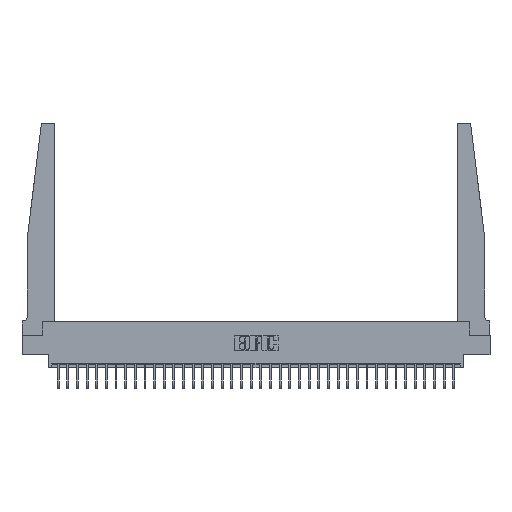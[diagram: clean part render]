
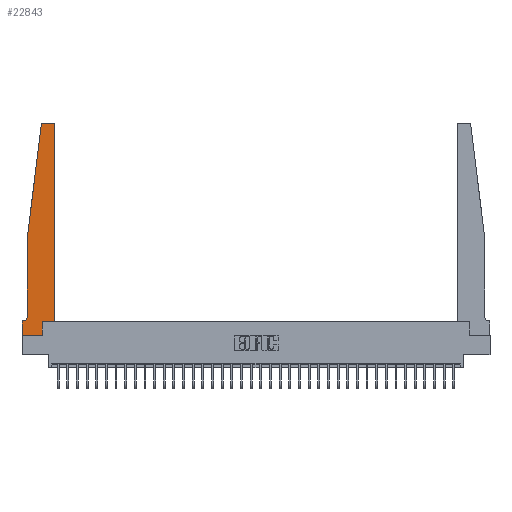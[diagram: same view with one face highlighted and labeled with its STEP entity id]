
A CAD part, top view. The second image highlights one B-rep face of the part: STEP entity #22843.
In plain terms, the highlighted planar face has unit normal (0, 0, 1).
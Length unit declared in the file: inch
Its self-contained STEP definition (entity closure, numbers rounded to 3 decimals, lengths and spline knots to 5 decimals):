
#201 = VECTOR ( 'NONE', #10803, 39.37008 ) ;
#574 = ORIENTED_EDGE ( 'NONE', *, *, #1850, .T. ) ;
#612 = CARTESIAN_POINT ( 'NONE',  ( 0., 0.1875, 0.37 ) ) ;
#661 = VERTEX_POINT ( 'NONE', #26374 ) ;
#939 = EDGE_CURVE ( 'NONE', #25772, #4605, #27736, .T. ) ;
#1061 = VECTOR ( 'NONE', #14592, 39.37008 ) ;
#1391 = DIRECTION ( 'NONE',  ( -0.122, -0.992, 0. ) ) ;
#1759 = LINE ( 'NONE', #13193, #201 ) ;
#1850 = EDGE_CURVE ( 'NONE', #4605, #10589, #10874, .T. ) ;
#2336 = VERTEX_POINT ( 'NONE', #3554 ) ;
#2435 = CARTESIAN_POINT ( 'NONE',  ( 0.425, 2.72, 0.37 ) ) ;
#2835 = CARTESIAN_POINT ( 'NONE',  ( 0.2605, 0., 0.37 ) ) ;
#2885 = AXIS2_PLACEMENT_3D ( 'NONE', #16379, #8387, #9315 ) ;
#3554 = CARTESIAN_POINT ( 'NONE',  ( 0., 0.1875, 0.37 ) ) ;
#3616 = AXIS2_PLACEMENT_3D ( 'NONE', #612, #29419, #15110 ) ;
#4387 = CARTESIAN_POINT ( 'NONE',  ( 0.425, 0.18, 0.37 ) ) ;
#4605 = VERTEX_POINT ( 'NONE', #12611 ) ;
#4637 = EDGE_CURVE ( 'NONE', #10589, #21681, #5285, .T. ) ;
#5099 = ORIENTED_EDGE ( 'NONE', *, *, #11352, .T. ) ;
#5236 = VECTOR ( 'NONE', #1391, 39.37008 ) ;
#5285 = LINE ( 'NONE', #15131, #16559 ) ;
#6821 = DIRECTION ( 'NONE',  ( 1., 0., 0. ) ) ;
#7274 = EDGE_CURVE ( 'NONE', #15423, #25772, #1759, .T. ) ;
#7332 = DIRECTION ( 'NONE',  ( 0., 1., 0. ) ) ;
#7657 = ORIENTED_EDGE ( 'NONE', *, *, #19373, .T. ) ;
#7843 = EDGE_LOOP ( 'NONE', ( #12732, #8987, #574, #9527, #17764, #7657, #10773, #11296, #29044, #15401, #5099, #12752 ) ) ;
#8076 = CARTESIAN_POINT ( 'NONE',  ( 0., 0., 0.37 ) ) ;
#8387 = DIRECTION ( 'NONE',  ( 0., 0., 1. ) ) ;
#8396 = VECTOR ( 'NONE', #28229, 39.37008 ) ;
#8714 = CARTESIAN_POINT ( 'NONE',  ( 0.425, 0.18, 0.37 ) ) ;
#8987 = ORIENTED_EDGE ( 'NONE', *, *, #939, .T. ) ;
#9048 = LINE ( 'NONE', #8076, #21014 ) ;
#9315 = DIRECTION ( 'NONE',  ( 1., 0., 0. ) ) ;
#9527 = ORIENTED_EDGE ( 'NONE', *, *, #4637, .T. ) ;
#9696 = CARTESIAN_POINT ( 'NONE',  ( 0.065, 0.1875, 0.37 ) ) ;
#9762 = VECTOR ( 'NONE', #7332, 39.37008 ) ;
#10589 = VERTEX_POINT ( 'NONE', #15959 ) ;
#10747 = EDGE_CURVE ( 'NONE', #10831, #15423, #12923, .T. ) ;
#10773 = ORIENTED_EDGE ( 'NONE', *, *, #18360, .T. ) ;
#10803 = DIRECTION ( 'NONE',  ( -1., 0., 0. ) ) ;
#10831 = VERTEX_POINT ( 'NONE', #2435 ) ;
#10874 = LINE ( 'NONE', #25245, #5236 ) ;
#11259 = AXIS2_PLACEMENT_3D ( 'NONE', #14144, #30876, #16585 ) ;
#11296 = ORIENTED_EDGE ( 'NONE', *, *, #23495, .T. ) ;
#11330 = CARTESIAN_POINT ( 'NONE',  ( 0.015, 0.2375, 0.37 ) ) ;
#11352 = EDGE_CURVE ( 'NONE', #18497, #10831, #20367, .T. ) ;
#12061 = CARTESIAN_POINT ( 'NONE',  ( 0.2605, 0.18, 0.37 ) ) ;
#12611 = CARTESIAN_POINT ( 'NONE',  ( 0.24675, 2.72367, 0.37 ) ) ;
#12732 = ORIENTED_EDGE ( 'NONE', *, *, #7274, .T. ) ;
#12752 = ORIENTED_EDGE ( 'NONE', *, *, #10747, .T. ) ;
#12923 = CIRCLE ( 'NONE', #11259, 0.03 ) ;
#13193 = CARTESIAN_POINT ( 'NONE',  ( 0.25, 2.75, 0.37 ) ) ;
#13413 = CARTESIAN_POINT ( 'NONE',  ( 0.27653, 2.75, 0.37 ) ) ;
#13713 = DIRECTION ( 'NONE',  ( -1., 0., 0. ) ) ;
#13905 = CARTESIAN_POINT ( 'NONE',  ( 0.425, 0.18, 0.37 ) ) ;
#14144 = CARTESIAN_POINT ( 'NONE',  ( 0.395, 2.72, 0.37 ) ) ;
#14592 = DIRECTION ( 'NONE',  ( -1., 0., 0. ) ) ;
#14847 = CARTESIAN_POINT ( 'NONE',  ( 0.065, 0.2375, 0.37 ) ) ;
#15110 = DIRECTION ( 'NONE',  ( 1., 0., 0. ) ) ;
#15131 = CARTESIAN_POINT ( 'NONE',  ( 0.065, 1.25, 0.37 ) ) ;
#15298 = DIRECTION ( 'NONE',  ( 0., -1., 0. ) ) ;
#15401 = ORIENTED_EDGE ( 'NONE', *, *, #16557, .T. ) ;
#15423 = VERTEX_POINT ( 'NONE', #23935 ) ;
#15959 = CARTESIAN_POINT ( 'NONE',  ( 0.065, 1.25, 0.37 ) ) ;
#16127 = VERTEX_POINT ( 'NONE', #2835 ) ;
#16379 = CARTESIAN_POINT ( 'NONE',  ( 0.27653, 2.72, 0.37 ) ) ;
#16467 = EDGE_CURVE ( 'NONE', #21681, #661, #29424, .T. ) ;
#16557 = EDGE_CURVE ( 'NONE', #19969, #18497, #28678, .T. ) ;
#16559 = VECTOR ( 'NONE', #17546, 39.37008 ) ;
#16585 = DIRECTION ( 'NONE',  ( 1., 0., 0. ) ) ;
#17032 = VERTEX_POINT ( 'NONE', #25702 ) ;
#17107 = LINE ( 'NONE', #29488, #22697 ) ;
#17546 = DIRECTION ( 'NONE',  ( 0., -1., 0. ) ) ;
#17764 = ORIENTED_EDGE ( 'NONE', *, *, #16467, .T. ) ;
#18360 = EDGE_CURVE ( 'NONE', #2336, #17032, #9048, .T. ) ;
#18497 = VERTEX_POINT ( 'NONE', #8714 ) ;
#18782 = EDGE_CURVE ( 'NONE', #16127, #19969, #21730, .T. ) ;
#18917 = FACE_OUTER_BOUND ( 'NONE', #7843, .T. ) ;
#19349 = VECTOR ( 'NONE', #6821, 39.37008 ) ;
#19373 = EDGE_CURVE ( 'NONE', #661, #2336, #25043, .T. ) ;
#19773 = AXIS2_PLACEMENT_3D ( 'NONE', #11330, #28028, #13713 ) ;
#19969 = VERTEX_POINT ( 'NONE', #12061 ) ;
#20367 = LINE ( 'NONE', #13905, #8396 ) ;
#21014 = VECTOR ( 'NONE', #15298, 39.37008 ) ;
#21650 = CARTESIAN_POINT ( 'NONE',  ( 0.2605, 0.18, 0.37 ) ) ;
#21681 = VERTEX_POINT ( 'NONE', #14847 ) ;
#21730 = LINE ( 'NONE', #21650, #9762 ) ;
#22697 = VECTOR ( 'NONE', #24676, 39.37008 ) ;
#22843 = ADVANCED_FACE ( 'NONE', ( #18917 ), #24609, .T. ) ;
#23495 = EDGE_CURVE ( 'NONE', #17032, #16127, #17107, .T. ) ;
#23935 = CARTESIAN_POINT ( 'NONE',  ( 0.395, 2.75, 0.37 ) ) ;
#24609 = PLANE ( 'NONE',  #3616 ) ;
#24676 = DIRECTION ( 'NONE',  ( 1., 0., 0. ) ) ;
#25043 = LINE ( 'NONE', #9696, #1061 ) ;
#25245 = CARTESIAN_POINT ( 'NONE',  ( 0.065, 1.25, 0.37 ) ) ;
#25702 = CARTESIAN_POINT ( 'NONE',  ( 0., 0., 0.37 ) ) ;
#25772 = VERTEX_POINT ( 'NONE', #13413 ) ;
#26374 = CARTESIAN_POINT ( 'NONE',  ( 0.015, 0.1875, 0.37 ) ) ;
#27736 = CIRCLE ( 'NONE', #2885, 0.03 ) ;
#28028 = DIRECTION ( 'NONE',  ( 0., 0., -1. ) ) ;
#28229 = DIRECTION ( 'NONE',  ( 0., 1., 0. ) ) ;
#28678 = LINE ( 'NONE', #4387, #19349 ) ;
#29044 = ORIENTED_EDGE ( 'NONE', *, *, #18782, .T. ) ;
#29419 = DIRECTION ( 'NONE',  ( 0., 0., 1. ) ) ;
#29424 = CIRCLE ( 'NONE', #19773, 0.05 ) ;
#29488 = CARTESIAN_POINT ( 'NONE',  ( 0., 0., 0.37 ) ) ;
#30876 = DIRECTION ( 'NONE',  ( 0., 0., 1. ) ) ;
